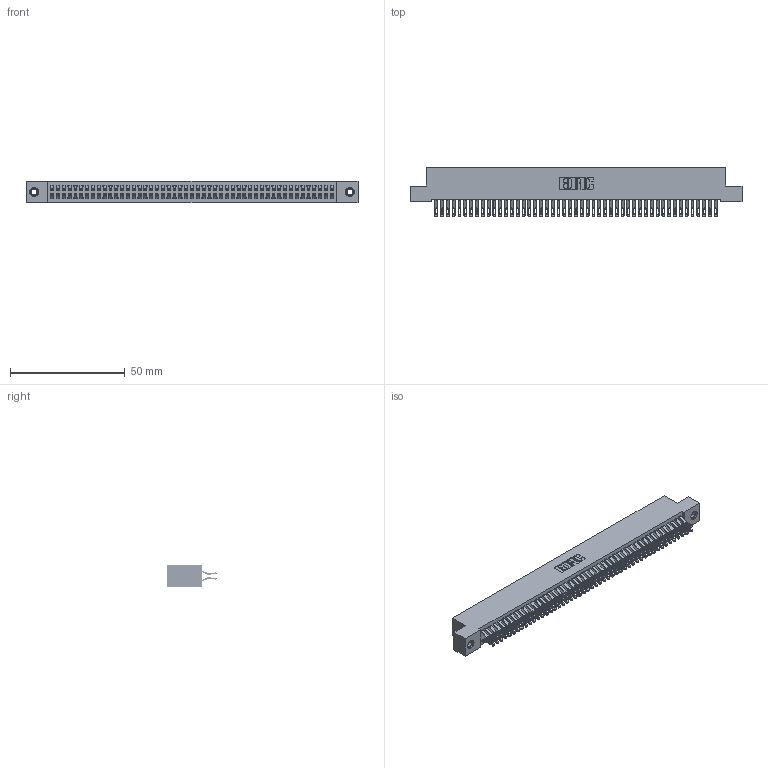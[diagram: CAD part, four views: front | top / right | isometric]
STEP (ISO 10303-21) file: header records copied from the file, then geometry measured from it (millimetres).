
FILE_DESCRIPTION (( 'STEP AP203' ), '1' );
FILE_NAME ('342-098-555-207.STEP', '2019-10-04T16:53:46', ( '' ), ( '' ), 'SwSTEP 2.0', 'SolidWorks 2016', '' );
FILE_SCHEMA (( 'CONFIG_CONTROL_DESIGN' ));
Length unit declared in the file: inch
Products named in the file (4): 345-250-001_345-250-005-103; 342-098-555-207; 342 Part_TI; 345-292-001_555 Tail
Assembly tree (101 placements, depth 2):
  342-098-555-207
    342 Part_TI
    345-292-001_555 Tail  x98
    345-250-001_345-250-005-103  x2
Bounding box: 144.78 x 21.47 x 9.4 mm (x, y, z)
Volume: 13301.3 mm3; surface area: 22797.6 mm2
Topology: 101 solids, 101 shells, 5854 faces, 18369 edges, 12238 vertices
Faces by surface type: plane 3430, cylinder 2408, cone 12, torus 4
Entity records: 31998 total; most frequent: CARTESIAN_POINT 5311, ORIENTED_EDGE 5210, DIRECTION 4527, EDGE_CURVE 2605, VECTOR 2437, LINE 2437, VERTEX_POINT 1732, AXIS2_PLACEMENT_3D 1045
